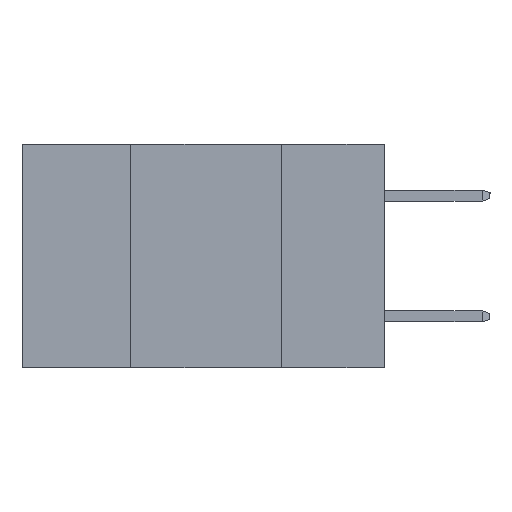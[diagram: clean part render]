
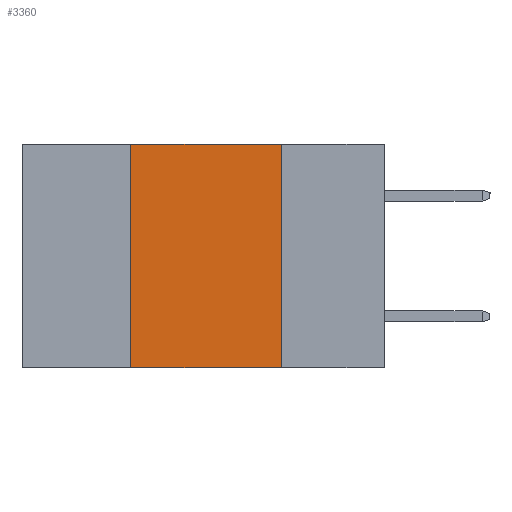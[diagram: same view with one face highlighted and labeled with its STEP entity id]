
A CAD part, left-side view. The second image highlights one B-rep face of the part: STEP entity #3360.
In plain terms, the highlighted planar face has unit normal (-1, 0, 0).
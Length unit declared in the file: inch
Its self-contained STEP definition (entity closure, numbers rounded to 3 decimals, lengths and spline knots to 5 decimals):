
#883 = FACE_OUTER_BOUND ( 'NONE', #2129, .T. ) ;
#894 = EDGE_CURVE ( 'NONE', #8605, #7495, #19110, .T. ) ;
#1832 = VECTOR ( 'NONE', #15227, 39.37008 ) ;
#1956 = VECTOR ( 'NONE', #16934, 39.37008 ) ;
#2129 = EDGE_LOOP ( 'NONE', ( #18441, #6706, #17159, #2513 ) ) ;
#2513 = ORIENTED_EDGE ( 'NONE', *, *, #894, .T. ) ;
#2899 = DIRECTION ( 'NONE',  ( 0., -1., 0. ) ) ;
#3360 = ADVANCED_FACE ( 'NONE', ( #883 ), #6814, .F. ) ;
#4067 = EDGE_CURVE ( 'NONE', #8605, #14171, #7651, .T. ) ;
#4798 = CARTESIAN_POINT ( 'NONE',  ( 0., 0.17, -0.37 ) ) ;
#5359 = DIRECTION ( 'NONE',  ( 1., 0., 0. ) ) ;
#6435 = CARTESIAN_POINT ( 'NONE',  ( 0., 0.6, 0. ) ) ;
#6706 = ORIENTED_EDGE ( 'NONE', *, *, #10861, .F. ) ;
#6814 = PLANE ( 'NONE',  #17605 ) ;
#7495 = VERTEX_POINT ( 'NONE', #10025 ) ;
#7606 = LINE ( 'NONE', #4798, #17174 ) ;
#7651 = LINE ( 'NONE', #18144, #1832 ) ;
#7676 = VERTEX_POINT ( 'NONE', #11383 ) ;
#8605 = VERTEX_POINT ( 'NONE', #19000 ) ;
#8662 = CARTESIAN_POINT ( 'NONE',  ( 0., 0.42, 0. ) ) ;
#10025 = CARTESIAN_POINT ( 'NONE',  ( 0., 0.17, -0.37 ) ) ;
#10861 = EDGE_CURVE ( 'NONE', #14171, #7676, #12200, .T. ) ;
#11281 = DIRECTION ( 'NONE',  ( 0., 0., -1. ) ) ;
#11383 = CARTESIAN_POINT ( 'NONE',  ( 0., 0.17, 0. ) ) ;
#11736 = CARTESIAN_POINT ( 'NONE',  ( 0., 0.6, -0.37 ) ) ;
#12200 = LINE ( 'NONE', #6435, #1956 ) ;
#12678 = VECTOR ( 'NONE', #2899, 39.37008 ) ;
#12750 = CARTESIAN_POINT ( 'NONE',  ( 0., 0.6, 0. ) ) ;
#13831 = EDGE_CURVE ( 'NONE', #7676, #7495, #7606, .T. ) ;
#14171 = VERTEX_POINT ( 'NONE', #8662 ) ;
#15227 = DIRECTION ( 'NONE',  ( 0., 0., 1. ) ) ;
#15289 = DIRECTION ( 'NONE',  ( 0., 0., -1. ) ) ;
#16934 = DIRECTION ( 'NONE',  ( 0., -1., 0. ) ) ;
#17159 = ORIENTED_EDGE ( 'NONE', *, *, #4067, .F. ) ;
#17174 = VECTOR ( 'NONE', #15289, 39.37008 ) ;
#17605 = AXIS2_PLACEMENT_3D ( 'NONE', #12750, #5359, #11281 ) ;
#18144 = CARTESIAN_POINT ( 'NONE',  ( 0., 0.42, -0.37 ) ) ;
#18441 = ORIENTED_EDGE ( 'NONE', *, *, #13831, .F. ) ;
#19000 = CARTESIAN_POINT ( 'NONE',  ( 0., 0.42, -0.37 ) ) ;
#19110 = LINE ( 'NONE', #11736, #12678 ) ;
